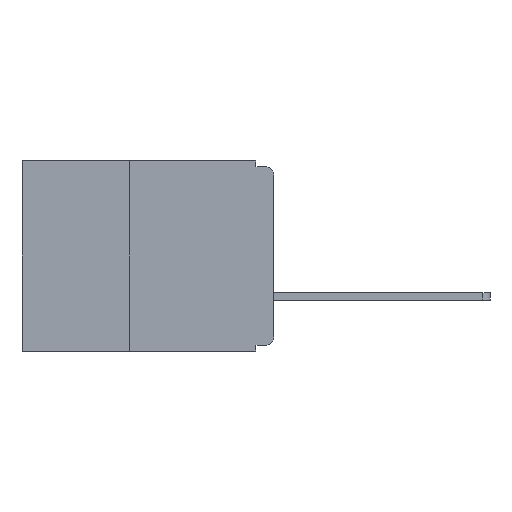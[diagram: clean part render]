
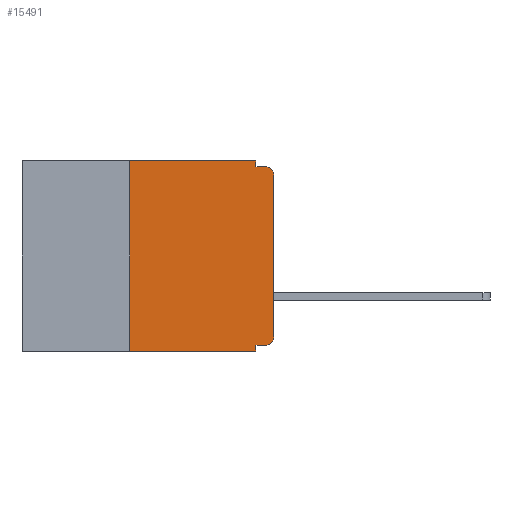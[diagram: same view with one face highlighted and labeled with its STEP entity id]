
A CAD part, left-side view. The second image highlights one B-rep face of the part: STEP entity #15491.
In plain terms, the highlighted planar face has unit normal (-1, 0, 0).
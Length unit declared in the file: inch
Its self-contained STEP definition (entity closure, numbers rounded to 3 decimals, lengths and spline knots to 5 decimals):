
#46 = VECTOR ( 'NONE', #19154, 39.37008 ) ;
#310 = DIRECTION ( 'NONE',  ( 0., 1., 0. ) ) ;
#388 = CARTESIAN_POINT ( 'NONE',  ( 0., 0., -0.32 ) ) ;
#403 = AXIS2_PLACEMENT_3D ( 'NONE', #7905, #22203, #10032 ) ;
#483 = LINE ( 'NONE', #388, #5424 ) ;
#719 = LINE ( 'NONE', #6796, #46 ) ;
#985 = ORIENTED_EDGE ( 'NONE', *, *, #1220, .T. ) ;
#1220 = EDGE_CURVE ( 'NONE', #15790, #16389, #4767, .T. ) ;
#1549 = VERTEX_POINT ( 'NONE', #17971 ) ;
#1613 = PLANE ( 'NONE',  #403 ) ;
#1795 = VERTEX_POINT ( 'NONE', #19123 ) ;
#1962 = CARTESIAN_POINT ( 'NONE',  ( 0., 0.25, -0.33 ) ) ;
#2409 = EDGE_CURVE ( 'NONE', #14311, #5124, #19601, .T. ) ;
#2493 = CARTESIAN_POINT ( 'NONE',  ( 0., 0.015, -0.32 ) ) ;
#4599 = ORIENTED_EDGE ( 'NONE', *, *, #22927, .F. ) ;
#4767 = CIRCLE ( 'NONE', #7245, 0.015 ) ;
#5124 = VERTEX_POINT ( 'NONE', #25216 ) ;
#5185 = EDGE_CURVE ( 'NONE', #14311, #12659, #16907, .T. ) ;
#5424 = VECTOR ( 'NONE', #310, 39.37008 ) ;
#6213 = DIRECTION ( 'NONE',  ( 0., -1., 0. ) ) ;
#6452 = CARTESIAN_POINT ( 'NONE',  ( 0., 0.437, 0. ) ) ;
#6695 = AXIS2_PLACEMENT_3D ( 'NONE', #7017, #21349, #9090 ) ;
#6796 = CARTESIAN_POINT ( 'NONE',  ( 0., 0., 0. ) ) ;
#7017 = CARTESIAN_POINT ( 'NONE',  ( 0., 0.015, -0.305 ) ) ;
#7245 = AXIS2_PLACEMENT_3D ( 'NONE', #26345, #26470, #26445 ) ;
#7370 = LINE ( 'NONE', #6452, #23008 ) ;
#7905 = CARTESIAN_POINT ( 'NONE',  ( 0., 0.437, 0. ) ) ;
#8004 = EDGE_CURVE ( 'NONE', #1549, #8224, #18785, .T. ) ;
#8224 = VERTEX_POINT ( 'NONE', #22143 ) ;
#8457 = CARTESIAN_POINT ( 'NONE',  ( 0., 0., -0.01 ) ) ;
#8514 = DIRECTION ( 'NONE',  ( 0., -1., 0. ) ) ;
#8515 = ORIENTED_EDGE ( 'NONE', *, *, #2409, .T. ) ;
#9090 = DIRECTION ( 'NONE',  ( 0., 0., -1. ) ) ;
#9134 = FACE_OUTER_BOUND ( 'NONE', #20421, .T. ) ;
#9344 = CIRCLE ( 'NONE', #6695, 0.015 ) ;
#9533 = ORIENTED_EDGE ( 'NONE', *, *, #9615, .F. ) ;
#9615 = EDGE_CURVE ( 'NONE', #12219, #13532, #483, .T. ) ;
#10032 = DIRECTION ( 'NONE',  ( 0., 0., -1. ) ) ;
#10811 = ORIENTED_EDGE ( 'NONE', *, *, #22259, .F. ) ;
#12219 = VERTEX_POINT ( 'NONE', #2493 ) ;
#12252 = EDGE_CURVE ( 'NONE', #1795, #15790, #719, .T. ) ;
#12659 = VERTEX_POINT ( 'NONE', #14811 ) ;
#13110 = CARTESIAN_POINT ( 'NONE',  ( 0., 0., -0.025 ) ) ;
#13532 = VERTEX_POINT ( 'NONE', #13890 ) ;
#13890 = CARTESIAN_POINT ( 'NONE',  ( 0., 0.031, -0.32 ) ) ;
#14030 = VECTOR ( 'NONE', #26453, 39.37008 ) ;
#14311 = VERTEX_POINT ( 'NONE', #1962 ) ;
#14692 = DIRECTION ( 'NONE',  ( 0., -1., 0. ) ) ;
#14811 = CARTESIAN_POINT ( 'NONE',  ( 0., 0.25, 0. ) ) ;
#15036 = ORIENTED_EDGE ( 'NONE', *, *, #5185, .F. ) ;
#15289 = VECTOR ( 'NONE', #25884, 39.37008 ) ;
#15491 = ADVANCED_FACE ( 'NONE', ( #9134 ), #1613, .F. ) ;
#15790 = VERTEX_POINT ( 'NONE', #13110 ) ;
#15936 = CARTESIAN_POINT ( 'NONE',  ( 0., 0.031, -0.33 ) ) ;
#16026 = ORIENTED_EDGE ( 'NONE', *, *, #8004, .F. ) ;
#16389 = VERTEX_POINT ( 'NONE', #23019 ) ;
#16436 = CARTESIAN_POINT ( 'NONE',  ( 0., 0.437, -0.33 ) ) ;
#16907 = LINE ( 'NONE', #23562, #22232 ) ;
#17232 = ORIENTED_EDGE ( 'NONE', *, *, #12252, .T. ) ;
#17971 = CARTESIAN_POINT ( 'NONE',  ( 0., 0.031, 0. ) ) ;
#18087 = VECTOR ( 'NONE', #14692, 39.37008 ) ;
#18711 = LINE ( 'NONE', #8457, #18087 ) ;
#18785 = LINE ( 'NONE', #26194, #14030 ) ;
#19123 = CARTESIAN_POINT ( 'NONE',  ( 0., 0., -0.305 ) ) ;
#19154 = DIRECTION ( 'NONE',  ( 0., 0., 1. ) ) ;
#19601 = LINE ( 'NONE', #16436, #24203 ) ;
#20129 = ORIENTED_EDGE ( 'NONE', *, *, #26130, .F. ) ;
#20421 = EDGE_LOOP ( 'NONE', ( #17232, #985, #10811, #16026, #4599, #15036, #8515, #20129, #9533, #23515 ) ) ;
#21349 = DIRECTION ( 'NONE',  ( -1., 0., 0. ) ) ;
#22143 = CARTESIAN_POINT ( 'NONE',  ( 0., 0.031, -0.01 ) ) ;
#22203 = DIRECTION ( 'NONE',  ( 1., 0., 0. ) ) ;
#22232 = VECTOR ( 'NONE', #23711, 39.37008 ) ;
#22259 = EDGE_CURVE ( 'NONE', #8224, #16389, #18711, .T. ) ;
#22407 = EDGE_CURVE ( 'NONE', #12219, #1795, #9344, .T. ) ;
#22927 = EDGE_CURVE ( 'NONE', #12659, #1549, #7370, .T. ) ;
#23008 = VECTOR ( 'NONE', #8514, 39.37008 ) ;
#23019 = CARTESIAN_POINT ( 'NONE',  ( 0., 0.015, -0.01 ) ) ;
#23515 = ORIENTED_EDGE ( 'NONE', *, *, #22407, .T. ) ;
#23562 = CARTESIAN_POINT ( 'NONE',  ( 0., 0.25, -0.33 ) ) ;
#23711 = DIRECTION ( 'NONE',  ( 0., 0., 1. ) ) ;
#24203 = VECTOR ( 'NONE', #6213, 39.37008 ) ;
#25216 = CARTESIAN_POINT ( 'NONE',  ( 0., 0.031, -0.33 ) ) ;
#25840 = LINE ( 'NONE', #15936, #15289 ) ;
#25884 = DIRECTION ( 'NONE',  ( 0., 0., -1. ) ) ;
#26130 = EDGE_CURVE ( 'NONE', #13532, #5124, #25840, .T. ) ;
#26194 = CARTESIAN_POINT ( 'NONE',  ( 0., 0.031, 0. ) ) ;
#26345 = CARTESIAN_POINT ( 'NONE',  ( 0., 0.015, -0.025 ) ) ;
#26445 = DIRECTION ( 'NONE',  ( 0., 0., -1. ) ) ;
#26453 = DIRECTION ( 'NONE',  ( 0., 0., -1. ) ) ;
#26470 = DIRECTION ( 'NONE',  ( -1., 0., 0. ) ) ;
